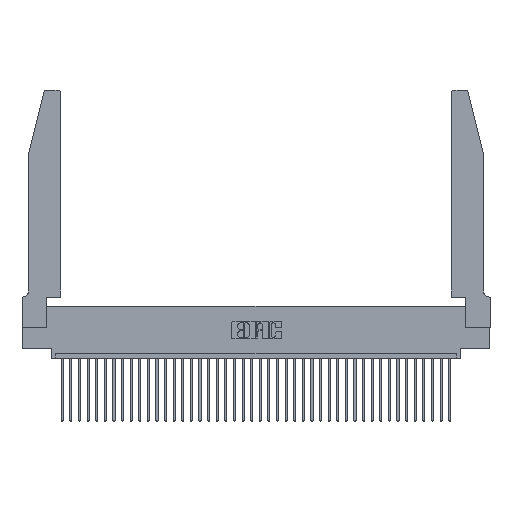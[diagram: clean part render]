
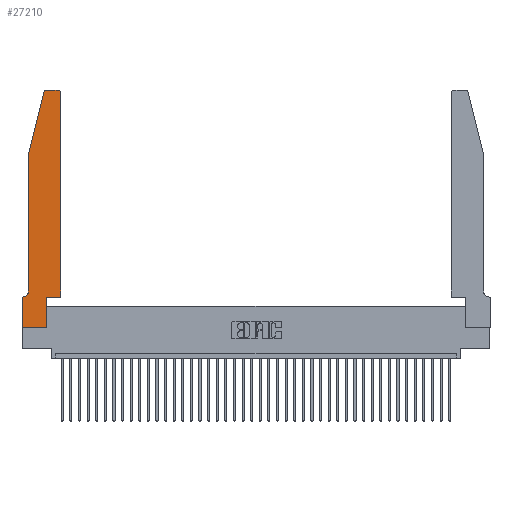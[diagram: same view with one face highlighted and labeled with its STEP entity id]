
A CAD part, top view. The second image highlights one B-rep face of the part: STEP entity #27210.
In plain terms, the highlighted planar face has unit normal (0, 0, 1).
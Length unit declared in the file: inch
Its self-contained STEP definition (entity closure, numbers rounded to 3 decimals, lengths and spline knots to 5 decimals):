
#205 = VECTOR ( 'NONE', #5337, 39.37008 ) ;
#288 = CARTESIAN_POINT ( 'NONE',  ( 0.284, 2.75, 0.37 ) ) ;
#631 = DIRECTION ( 'NONE',  ( 0., -1., 0. ) ) ;
#1344 = CIRCLE ( 'NONE', #6762, 0.03 ) ;
#1650 = CARTESIAN_POINT ( 'NONE',  ( 0.0755, 2., 0.37 ) ) ;
#2467 = VERTEX_POINT ( 'NONE', #20606 ) ;
#2803 = LINE ( 'NONE', #27686, #36667 ) ;
#3730 = CARTESIAN_POINT ( 'NONE',  ( 0.0055, 0.35, 0.37 ) ) ;
#3835 = EDGE_CURVE ( 'NONE', #8834, #24257, #1344, .T. ) ;
#3862 = VERTEX_POINT ( 'NONE', #37673 ) ;
#4305 = AXIS2_PLACEMENT_3D ( 'NONE', #28918, #16600, #10343 ) ;
#4423 = CARTESIAN_POINT ( 'NONE',  ( 0.0755, 0.35, 0.37 ) ) ;
#4770 = DIRECTION ( 'NONE',  ( 1., 0., 0. ) ) ;
#4789 = LINE ( 'NONE', #38132, #7619 ) ;
#5026 = VECTOR ( 'NONE', #30057, 39.37008 ) ;
#5132 = ORIENTED_EDGE ( 'NONE', *, *, #17256, .T. ) ;
#5337 = DIRECTION ( 'NONE',  ( -1., 0., 0. ) ) ;
#5515 = VECTOR ( 'NONE', #24873, 39.37008 ) ;
#5772 = LINE ( 'NONE', #29455, #36787 ) ;
#6244 = DIRECTION ( 'NONE',  ( -1., 0., 0. ) ) ;
#6347 = VERTEX_POINT ( 'NONE', #31797 ) ;
#6762 = AXIS2_PLACEMENT_3D ( 'NONE', #22157, #28258, #34498 ) ;
#6780 = EDGE_CURVE ( 'NONE', #13081, #31967, #7123, .T. ) ;
#7123 = CIRCLE ( 'NONE', #4305, 0.03 ) ;
#7619 = VECTOR ( 'NONE', #23184, 39.37008 ) ;
#8768 = DIRECTION ( 'NONE',  ( -1., 0., 0. ) ) ;
#8817 = LINE ( 'NONE', #22266, #5515 ) ;
#8834 = VERTEX_POINT ( 'NONE', #288 ) ;
#10343 = DIRECTION ( 'NONE',  ( 1., 0., 0. ) ) ;
#10496 = VECTOR ( 'NONE', #25075, 39.37008 ) ;
#10890 = VERTEX_POINT ( 'NONE', #23525 ) ;
#11230 = AXIS2_PLACEMENT_3D ( 'NONE', #35241, #14366, #4770 ) ;
#11386 = PLANE ( 'NONE',  #11230 ) ;
#11916 = EDGE_CURVE ( 'NONE', #24257, #3862, #5772, .T. ) ;
#12088 = EDGE_CURVE ( 'NONE', #28620, #30880, #38246, .T. ) ;
#13081 = VERTEX_POINT ( 'NONE', #26351 ) ;
#14366 = DIRECTION ( 'NONE',  ( 0., 0., 1. ) ) ;
#16595 = EDGE_CURVE ( 'NONE', #6347, #28620, #8817, .T. ) ;
#16600 = DIRECTION ( 'NONE',  ( 0., 0., 1. ) ) ;
#16933 = CARTESIAN_POINT ( 'NONE',  ( 0.4505, 0.35, 0.37 ) ) ;
#17149 = DIRECTION ( 'NONE',  ( 0., -1., 0. ) ) ;
#17186 = LINE ( 'NONE', #4423, #205 ) ;
#17256 = EDGE_CURVE ( 'NONE', #30348, #10890, #17186, .T. ) ;
#18507 = CARTESIAN_POINT ( 'NONE',  ( 0.4205, 2.75, 0.37 ) ) ;
#18637 = ORIENTED_EDGE ( 'NONE', *, *, #3835, .T. ) ;
#18903 = CARTESIAN_POINT ( 'NONE',  ( 0.2865, 0.35, 0.37 ) ) ;
#20457 = ORIENTED_EDGE ( 'NONE', *, *, #11916, .T. ) ;
#20578 = CARTESIAN_POINT ( 'NONE',  ( 0.0055, 0.42, 0.37 ) ) ;
#20601 = CARTESIAN_POINT ( 'NONE',  ( 0.25487, 2.72718, 0.37 ) ) ;
#20606 = CARTESIAN_POINT ( 'NONE',  ( 0.0755, 0.42, 0.37 ) ) ;
#21021 = LINE ( 'NONE', #33142, #5026 ) ;
#21173 = VECTOR ( 'NONE', #17149, 39.37008 ) ;
#21614 = ORIENTED_EDGE ( 'NONE', *, *, #12088, .T. ) ;
#21758 = CARTESIAN_POINT ( 'NONE',  ( 0.4505, 0.35, 0.37 ) ) ;
#22157 = CARTESIAN_POINT ( 'NONE',  ( 0.284, 2.72, 0.37 ) ) ;
#22266 = CARTESIAN_POINT ( 'NONE',  ( 0.2865, 0.35, 0.37 ) ) ;
#23184 = DIRECTION ( 'NONE',  ( 0., 1., 0. ) ) ;
#23264 = DIRECTION ( 'NONE',  ( 0., 0., -1. ) ) ;
#23525 = CARTESIAN_POINT ( 'NONE',  ( 0., 0.35, 0.37 ) ) ;
#23831 = ORIENTED_EDGE ( 'NONE', *, *, #36326, .T. ) ;
#24257 = VERTEX_POINT ( 'NONE', #20601 ) ;
#24415 = CARTESIAN_POINT ( 'NONE',  ( 0.2605, 2.75, 0.37 ) ) ;
#24873 = DIRECTION ( 'NONE',  ( 0., 1., 0. ) ) ;
#25075 = DIRECTION ( 'NONE',  ( 1., 0., 0. ) ) ;
#25148 = CARTESIAN_POINT ( 'NONE',  ( 0., 0., 0.37 ) ) ;
#25345 = VECTOR ( 'NONE', #6244, 39.37008 ) ;
#25497 = ORIENTED_EDGE ( 'NONE', *, *, #36923, .T. ) ;
#25656 = ORIENTED_EDGE ( 'NONE', *, *, #6780, .T. ) ;
#26351 = CARTESIAN_POINT ( 'NONE',  ( 0.4505, 2.72, 0.37 ) ) ;
#26466 = CIRCLE ( 'NONE', #38442, 0.07 ) ;
#27210 = ADVANCED_FACE ( 'NONE', ( #28121 ), #11386, .T. ) ;
#27686 = CARTESIAN_POINT ( 'NONE',  ( 0., 0., 0.37 ) ) ;
#28121 = FACE_OUTER_BOUND ( 'NONE', #38365, .T. ) ;
#28258 = DIRECTION ( 'NONE',  ( 0., 0., 1. ) ) ;
#28620 = VERTEX_POINT ( 'NONE', #18903 ) ;
#28918 = CARTESIAN_POINT ( 'NONE',  ( 0.4205, 2.72, 0.37 ) ) ;
#29455 = CARTESIAN_POINT ( 'NONE',  ( 0.0755, 2., 0.37 ) ) ;
#29892 = EDGE_CURVE ( 'NONE', #2467, #30348, #26466, .T. ) ;
#29951 = ORIENTED_EDGE ( 'NONE', *, *, #16595, .T. ) ;
#30057 = DIRECTION ( 'NONE',  ( 1., 0., 0. ) ) ;
#30163 = ORIENTED_EDGE ( 'NONE', *, *, #35075, .T. ) ;
#30196 = ORIENTED_EDGE ( 'NONE', *, *, #34435, .T. ) ;
#30348 = VERTEX_POINT ( 'NONE', #3730 ) ;
#30880 = VERTEX_POINT ( 'NONE', #16933 ) ;
#31027 = ORIENTED_EDGE ( 'NONE', *, *, #29892, .T. ) ;
#31797 = CARTESIAN_POINT ( 'NONE',  ( 0.2865, 0., 0.37 ) ) ;
#31967 = VERTEX_POINT ( 'NONE', #18507 ) ;
#32249 = VERTEX_POINT ( 'NONE', #25148 ) ;
#33142 = CARTESIAN_POINT ( 'NONE',  ( 0., 0., 0.37 ) ) ;
#34435 = EDGE_CURVE ( 'NONE', #30880, #13081, #4789, .T. ) ;
#34498 = DIRECTION ( 'NONE',  ( 1., 0., 0. ) ) ;
#35075 = EDGE_CURVE ( 'NONE', #3862, #2467, #37181, .T. ) ;
#35241 = CARTESIAN_POINT ( 'NONE',  ( 0., 0.35, 0.37 ) ) ;
#35353 = EDGE_CURVE ( 'NONE', #10890, #32249, #2803, .T. ) ;
#36326 = EDGE_CURVE ( 'NONE', #31967, #8834, #38992, .T. ) ;
#36667 = VECTOR ( 'NONE', #631, 39.37008 ) ;
#36787 = VECTOR ( 'NONE', #38472, 39.37008 ) ;
#36923 = EDGE_CURVE ( 'NONE', #32249, #6347, #21021, .T. ) ;
#37181 = LINE ( 'NONE', #1650, #21173 ) ;
#37673 = CARTESIAN_POINT ( 'NONE',  ( 0.0755, 2., 0.37 ) ) ;
#37966 = ORIENTED_EDGE ( 'NONE', *, *, #35353, .T. ) ;
#38132 = CARTESIAN_POINT ( 'NONE',  ( 0.4505, 0.35, 0.37 ) ) ;
#38246 = LINE ( 'NONE', #21758, #10496 ) ;
#38365 = EDGE_LOOP ( 'NONE', ( #23831, #18637, #20457, #30163, #31027, #5132, #37966, #25497, #29951, #21614, #30196, #25656 ) ) ;
#38442 = AXIS2_PLACEMENT_3D ( 'NONE', #20578, #23264, #8768 ) ;
#38472 = DIRECTION ( 'NONE',  ( -0.239, -0.971, 0. ) ) ;
#38992 = LINE ( 'NONE', #24415, #25345 ) ;
